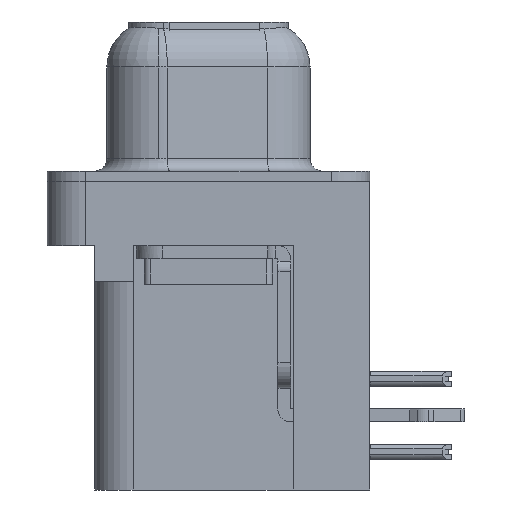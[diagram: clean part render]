
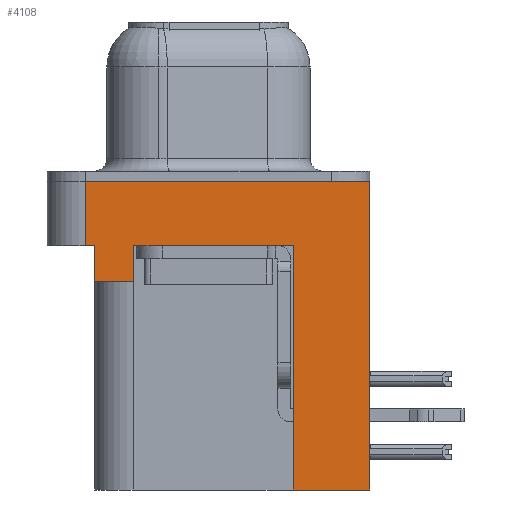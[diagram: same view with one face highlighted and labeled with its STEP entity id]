
A CAD part, left-side view. The second image highlights one B-rep face of the part: STEP entity #4108.
In plain terms, the highlighted planar face has unit normal (-1, 0, 0).
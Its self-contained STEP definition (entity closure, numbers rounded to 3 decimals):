
#314 = VECTOR ( 'NONE', #10906, 1000. ) ;
#368 = CARTESIAN_POINT ( 'NONE',  ( -2.91, -6.275, -2.5 ) ) ;
#719 = AXIS2_PLACEMENT_3D ( 'NONE', #15535, #13649, #8555 ) ;
#846 = FACE_OUTER_BOUND ( 'NONE', #19544, .T. ) ;
#1065 = DIRECTION ( 'NONE',  ( 0., -1., 0. ) ) ;
#1205 = DIRECTION ( 'NONE',  ( 0., 0., 1. ) ) ;
#1486 = LINE ( 'NONE', #19614, #314 ) ;
#1919 = CARTESIAN_POINT ( 'NONE',  ( -2.91, 4.425, -3.9 ) ) ;
#3248 = CARTESIAN_POINT ( 'NONE',  ( -2.91, 2.895, -3.9 ) ) ;
#3349 = ORIENTED_EDGE ( 'NONE', *, *, #9344, .F. ) ;
#3510 = VECTOR ( 'NONE', #13325, 1000. ) ;
#4036 = VECTOR ( 'NONE', #19643, 1000. ) ;
#4108 = ADVANCED_FACE ( 'NONE', ( #846 ), #20717, .T. ) ;
#4225 = DIRECTION ( 'NONE',  ( 0., -1., 0. ) ) ;
#4334 = EDGE_CURVE ( 'NONE', #9491, #18281, #5385, .T. ) ;
#4406 = LINE ( 'NONE', #368, #8447 ) ;
#4899 = EDGE_CURVE ( 'NONE', #20189, #19485, #1486, .T. ) ;
#5121 = CARTESIAN_POINT ( 'NONE',  ( -2.91, 4.775, -2.5 ) ) ;
#5385 = LINE ( 'NONE', #17389, #4036 ) ;
#5472 = EDGE_CURVE ( 'NONE', #15289, #19485, #8433, .T. ) ;
#5564 = ORIENTED_EDGE ( 'NONE', *, *, #13469, .F. ) ;
#5946 = CARTESIAN_POINT ( 'NONE',  ( -2.91, -6.275, 0. ) ) ;
#6210 = CARTESIAN_POINT ( 'NONE',  ( -2.91, -3.295, -2.5 ) ) ;
#6385 = ORIENTED_EDGE ( 'NONE', *, *, #14236, .T. ) ;
#6480 = CARTESIAN_POINT ( 'NONE',  ( -2.91, 2.895, -3.9 ) ) ;
#7188 = VECTOR ( 'NONE', #21584, 1000. ) ;
#7532 = EDGE_CURVE ( 'NONE', #18581, #20189, #8892, .T. ) ;
#7582 = EDGE_CURVE ( 'NONE', #18581, #20178, #18306, .T. ) ;
#7733 = VECTOR ( 'NONE', #17994, 1000. ) ;
#7794 = CARTESIAN_POINT ( 'NONE',  ( -2.91, -6.275, -2.5 ) ) ;
#7922 = VERTEX_POINT ( 'NONE', #18186 ) ;
#8433 = LINE ( 'NONE', #7794, #12176 ) ;
#8447 = VECTOR ( 'NONE', #14104, 1000. ) ;
#8555 = DIRECTION ( 'NONE',  ( 0., 0., 1. ) ) ;
#8762 = CARTESIAN_POINT ( 'NONE',  ( -2.91, 2.895, -2.5 ) ) ;
#8892 = LINE ( 'NONE', #16712, #3510 ) ;
#9344 = EDGE_CURVE ( 'NONE', #13634, #7922, #12035, .T. ) ;
#9482 = EDGE_CURVE ( 'NONE', #18281, #20926, #9912, .T. ) ;
#9491 = VERTEX_POINT ( 'NONE', #16414 ) ;
#9912 = LINE ( 'NONE', #14673, #7188 ) ;
#10186 = ORIENTED_EDGE ( 'NONE', *, *, #9482, .F. ) ;
#10906 = DIRECTION ( 'NONE',  ( 0., 0., 1. ) ) ;
#12035 = LINE ( 'NONE', #5946, #7733 ) ;
#12176 = VECTOR ( 'NONE', #1065, 1000. ) ;
#12472 = LINE ( 'NONE', #14945, #15424 ) ;
#12608 = LINE ( 'NONE', #16193, #12885 ) ;
#12885 = VECTOR ( 'NONE', #4225, 1000. ) ;
#13325 = DIRECTION ( 'NONE',  ( 0., 1., 0. ) ) ;
#13359 = ORIENTED_EDGE ( 'NONE', *, *, #4334, .F. ) ;
#13469 = EDGE_CURVE ( 'NONE', #15289, #13634, #12472, .T. ) ;
#13634 = VERTEX_POINT ( 'NONE', #14014 ) ;
#13649 = DIRECTION ( 'NONE',  ( -1., 0., 0. ) ) ;
#14014 = CARTESIAN_POINT ( 'NONE',  ( -2.91, 4.775, 0. ) ) ;
#14104 = DIRECTION ( 'NONE',  ( 0., 0., 1. ) ) ;
#14236 = EDGE_CURVE ( 'NONE', #9491, #7922, #4406, .T. ) ;
#14541 = ORIENTED_EDGE ( 'NONE', *, *, #17044, .T. ) ;
#14673 = CARTESIAN_POINT ( 'NONE',  ( -2.91, -3.295, -12. ) ) ;
#14890 = ORIENTED_EDGE ( 'NONE', *, *, #7582, .T. ) ;
#14945 = CARTESIAN_POINT ( 'NONE',  ( -2.91, 4.775, -2.5 ) ) ;
#15072 = CARTESIAN_POINT ( 'NONE',  ( -2.91, 4.425, -2.5 ) ) ;
#15227 = CARTESIAN_POINT ( 'NONE',  ( -2.91, -3.295, -12. ) ) ;
#15289 = VERTEX_POINT ( 'NONE', #5121 ) ;
#15403 = ORIENTED_EDGE ( 'NONE', *, *, #5472, .T. ) ;
#15424 = VECTOR ( 'NONE', #1205, 1000. ) ;
#15535 = CARTESIAN_POINT ( 'NONE',  ( -2.91, -6.275, -2.5 ) ) ;
#16193 = CARTESIAN_POINT ( 'NONE',  ( -2.91, -6.275, -2.5 ) ) ;
#16414 = CARTESIAN_POINT ( 'NONE',  ( -2.91, -6.275, -12. ) ) ;
#16712 = CARTESIAN_POINT ( 'NONE',  ( -2.91, 4.425, -3.9 ) ) ;
#17044 = EDGE_CURVE ( 'NONE', #20178, #20926, #12608, .T. ) ;
#17389 = CARTESIAN_POINT ( 'NONE',  ( -2.91, -3.295, -12. ) ) ;
#17468 = VECTOR ( 'NONE', #22095, 1000. ) ;
#17994 = DIRECTION ( 'NONE',  ( 0., -1., 0. ) ) ;
#18186 = CARTESIAN_POINT ( 'NONE',  ( -2.91, -6.275, 0. ) ) ;
#18281 = VERTEX_POINT ( 'NONE', #15227 ) ;
#18306 = LINE ( 'NONE', #3248, #17468 ) ;
#18581 = VERTEX_POINT ( 'NONE', #6480 ) ;
#18958 = ORIENTED_EDGE ( 'NONE', *, *, #7532, .F. ) ;
#19485 = VERTEX_POINT ( 'NONE', #15072 ) ;
#19544 = EDGE_LOOP ( 'NONE', ( #3349, #5564, #15403, #21797, #18958, #14890, #14541, #10186, #13359, #6385 ) ) ;
#19614 = CARTESIAN_POINT ( 'NONE',  ( -2.91, 4.425, -3.9 ) ) ;
#19643 = DIRECTION ( 'NONE',  ( 0., 1., 0. ) ) ;
#20178 = VERTEX_POINT ( 'NONE', #8762 ) ;
#20189 = VERTEX_POINT ( 'NONE', #1919 ) ;
#20717 = PLANE ( 'NONE',  #719 ) ;
#20926 = VERTEX_POINT ( 'NONE', #6210 ) ;
#21584 = DIRECTION ( 'NONE',  ( 0., 0., 1. ) ) ;
#21797 = ORIENTED_EDGE ( 'NONE', *, *, #4899, .F. ) ;
#22095 = DIRECTION ( 'NONE',  ( 0., 0., 1. ) ) ;
